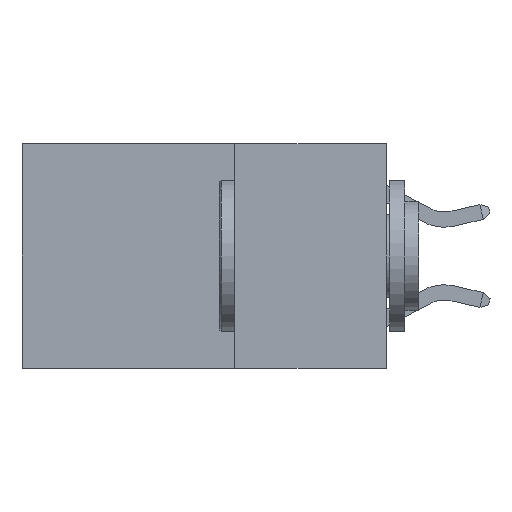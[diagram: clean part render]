
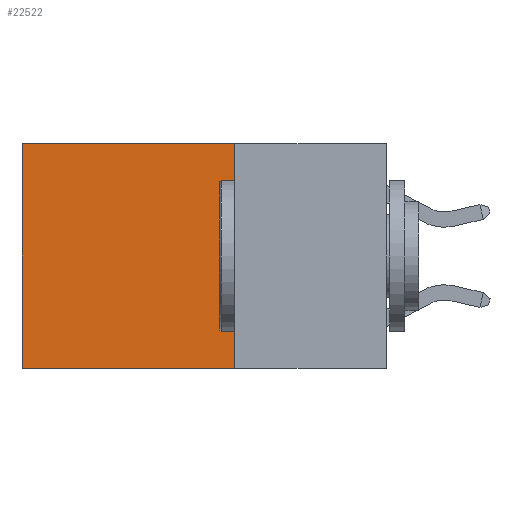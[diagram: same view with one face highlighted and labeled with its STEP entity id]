
A CAD part, left-side view. The second image highlights one B-rep face of the part: STEP entity #22522.
In plain terms, the highlighted planar face has unit normal (-1, 0, 0).
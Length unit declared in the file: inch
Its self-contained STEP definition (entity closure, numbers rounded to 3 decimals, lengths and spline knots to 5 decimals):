
#182 = EDGE_LOOP ( 'NONE', ( #11115, #22963, #16992, #11244 ) ) ;
#290 = CARTESIAN_POINT ( 'NONE',  ( 0.2625, 0.25, 0. ) ) ;
#1141 = AXIS2_PLACEMENT_3D ( 'NONE', #20279, #7644, #22380 ) ;
#2978 = DIRECTION ( 'NONE',  ( 0., 1., 0. ) ) ;
#6662 = LINE ( 'NONE', #8633, #22838 ) ;
#7110 = LINE ( 'NONE', #17398, #12082 ) ;
#7644 = DIRECTION ( 'NONE',  ( 1., 0., 0. ) ) ;
#8633 = CARTESIAN_POINT ( 'NONE',  ( 0.2625, 0.25, 0. ) ) ;
#10857 = VERTEX_POINT ( 'NONE', #16761 ) ;
#11079 = EDGE_CURVE ( 'NONE', #24009, #20668, #7110, .T. ) ;
#11115 = ORIENTED_EDGE ( 'NONE', *, *, #11079, .T. ) ;
#11244 = ORIENTED_EDGE ( 'NONE', *, *, #13904, .T. ) ;
#12082 = VECTOR ( 'NONE', #19503, 39.37008 ) ;
#12399 = EDGE_CURVE ( 'NONE', #10857, #15635, #26143, .T. ) ;
#12900 = FACE_OUTER_BOUND ( 'NONE', #182, .T. ) ;
#13004 = DIRECTION ( 'NONE',  ( 0., 0., -1. ) ) ;
#13198 = VECTOR ( 'NONE', #2978, 39.37008 ) ;
#13904 = EDGE_CURVE ( 'NONE', #10857, #24009, #6662, .T. ) ;
#15635 = VERTEX_POINT ( 'NONE', #20244 ) ;
#16761 = CARTESIAN_POINT ( 'NONE',  ( 0.2625, 0.25, 0. ) ) ;
#16992 = ORIENTED_EDGE ( 'NONE', *, *, #12399, .F. ) ;
#17398 = CARTESIAN_POINT ( 'NONE',  ( 0.2625, 0.6, 0. ) ) ;
#18094 = PLANE ( 'NONE',  #1141 ) ;
#19254 = EDGE_CURVE ( 'NONE', #15635, #20668, #25016, .T. ) ;
#19503 = DIRECTION ( 'NONE',  ( 0., 0., -1. ) ) ;
#20244 = CARTESIAN_POINT ( 'NONE',  ( 0.2625, 0.25, -0.37 ) ) ;
#20279 = CARTESIAN_POINT ( 'NONE',  ( 0.2625, 0.25, 0. ) ) ;
#20668 = VERTEX_POINT ( 'NONE', #26692 ) ;
#21264 = VECTOR ( 'NONE', #13004, 39.37008 ) ;
#21414 = DIRECTION ( 'NONE',  ( 0., 1., 0. ) ) ;
#22380 = DIRECTION ( 'NONE',  ( 0., 0., -1. ) ) ;
#22522 = ADVANCED_FACE ( 'NONE', ( #12900 ), #18094, .F. ) ;
#22838 = VECTOR ( 'NONE', #21414, 39.37008 ) ;
#22963 = ORIENTED_EDGE ( 'NONE', *, *, #19254, .F. ) ;
#23445 = CARTESIAN_POINT ( 'NONE',  ( 0.2625, 0.25, -0.37 ) ) ;
#24009 = VERTEX_POINT ( 'NONE', #24787 ) ;
#24787 = CARTESIAN_POINT ( 'NONE',  ( 0.2625, 0.6, 0. ) ) ;
#25016 = LINE ( 'NONE', #23445, #13198 ) ;
#26143 = LINE ( 'NONE', #290, #21264 ) ;
#26692 = CARTESIAN_POINT ( 'NONE',  ( 0.2625, 0.6, -0.37 ) ) ;
